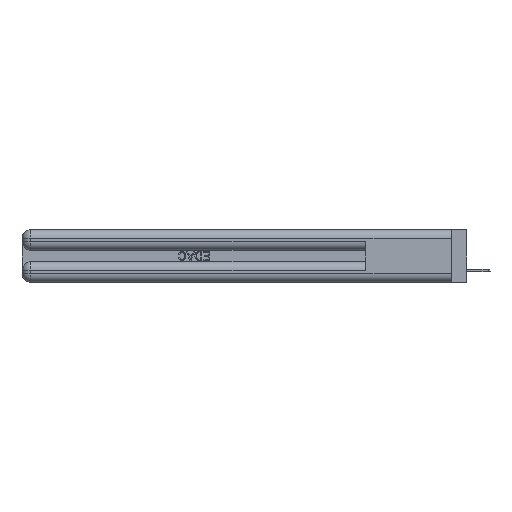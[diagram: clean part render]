
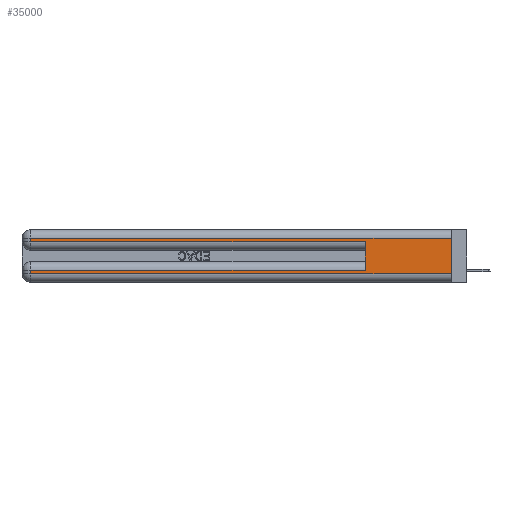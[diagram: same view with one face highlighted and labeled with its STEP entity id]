
A CAD part, left-side view. The second image highlights one B-rep face of the part: STEP entity #35000.
In plain terms, the highlighted planar face has unit normal (-1, 0, 0).
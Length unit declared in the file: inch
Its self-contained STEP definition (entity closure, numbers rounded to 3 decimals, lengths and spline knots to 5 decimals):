
#63 = ORIENTED_EDGE ( 'NONE', *, *, #6155, .F. ) ;
#1035 = DIRECTION ( 'NONE',  ( 0., -1., 0. ) ) ;
#2873 = FACE_OUTER_BOUND ( 'NONE', #14043, .T. ) ;
#3079 = DIRECTION ( 'NONE',  ( 0., 0., 1. ) ) ;
#4505 = LINE ( 'NONE', #20849, #42558 ) ;
#4718 = VERTEX_POINT ( 'NONE', #31403 ) ;
#4938 = LINE ( 'NONE', #20452, #36094 ) ;
#6155 = EDGE_CURVE ( 'NONE', #16280, #14997, #4505, .T. ) ;
#6618 = VERTEX_POINT ( 'NONE', #38588 ) ;
#6661 = CARTESIAN_POINT ( 'NONE',  ( 0., 0.6, 0.145 ) ) ;
#6908 = VERTEX_POINT ( 'NONE', #19527 ) ;
#7484 = LINE ( 'NONE', #41129, #29659 ) ;
#7557 = VECTOR ( 'NONE', #22286, 39.37008 ) ;
#7573 = LINE ( 'NONE', #6661, #22353 ) ;
#8105 = ORIENTED_EDGE ( 'NONE', *, *, #33060, .F. ) ;
#9645 = CARTESIAN_POINT ( 'NONE',  ( 0., 2.94, 0.085 ) ) ;
#10424 = DIRECTION ( 'NONE',  ( 1., 0., 0. ) ) ;
#10462 = CARTESIAN_POINT ( 'NONE',  ( 0., 0., 0.31 ) ) ;
#11125 = EDGE_CURVE ( 'NONE', #6908, #14997, #28765, .T. ) ;
#12103 = CARTESIAN_POINT ( 'NONE',  ( 0., 0., 0.31 ) ) ;
#14043 = EDGE_LOOP ( 'NONE', ( #63, #25486, #31046, #39941, #8105, #18049, #36142, #43435 ) ) ;
#14336 = CARTESIAN_POINT ( 'NONE',  ( 0., 2.94, 0.285 ) ) ;
#14997 = VERTEX_POINT ( 'NONE', #36721 ) ;
#16280 = VERTEX_POINT ( 'NONE', #10462 ) ;
#17372 = EDGE_CURVE ( 'NONE', #18128, #6908, #19222, .T. ) ;
#18049 = ORIENTED_EDGE ( 'NONE', *, *, #22112, .T. ) ;
#18128 = VERTEX_POINT ( 'NONE', #9645 ) ;
#19222 = LINE ( 'NONE', #38203, #41896 ) ;
#19527 = CARTESIAN_POINT ( 'NONE',  ( 0., 2.94, 0.06 ) ) ;
#20452 = CARTESIAN_POINT ( 'NONE',  ( 0., 2.94, 0.37 ) ) ;
#20581 = VERTEX_POINT ( 'NONE', #38969 ) ;
#20849 = CARTESIAN_POINT ( 'NONE',  ( 0., 0., 0.37 ) ) ;
#21319 = DIRECTION ( 'NONE',  ( 0., -1., 0. ) ) ;
#22112 = EDGE_CURVE ( 'NONE', #4718, #18128, #7484, .T. ) ;
#22286 = DIRECTION ( 'NONE',  ( 0., 1., 0. ) ) ;
#22353 = VECTOR ( 'NONE', #3079, 39.37008 ) ;
#22427 = VECTOR ( 'NONE', #1035, 39.37008 ) ;
#24831 = DIRECTION ( 'NONE',  ( 0., 0., -1. ) ) ;
#25486 = ORIENTED_EDGE ( 'NONE', *, *, #36674, .T. ) ;
#26225 = EDGE_CURVE ( 'NONE', #6618, #30972, #4938, .T. ) ;
#26374 = EDGE_CURVE ( 'NONE', #30972, #20581, #29264, .T. ) ;
#27460 = CARTESIAN_POINT ( 'NONE',  ( 0., 0., 0.06 ) ) ;
#28765 = LINE ( 'NONE', #27460, #22427 ) ;
#29264 = LINE ( 'NONE', #31600, #39817 ) ;
#29659 = VECTOR ( 'NONE', #40976, 39.37008 ) ;
#30433 = CARTESIAN_POINT ( 'NONE',  ( 0., 0., 0.37 ) ) ;
#30968 = DIRECTION ( 'NONE',  ( 0., 0., -1. ) ) ;
#30972 = VERTEX_POINT ( 'NONE', #14336 ) ;
#31046 = ORIENTED_EDGE ( 'NONE', *, *, #26225, .T. ) ;
#31403 = CARTESIAN_POINT ( 'NONE',  ( 0., 0.6, 0.085 ) ) ;
#31600 = CARTESIAN_POINT ( 'NONE',  ( 0., 0., 0.285 ) ) ;
#33060 = EDGE_CURVE ( 'NONE', #4718, #20581, #7573, .T. ) ;
#33829 = PLANE ( 'NONE',  #39838 ) ;
#33992 = DIRECTION ( 'NONE',  ( 0., 0., -1. ) ) ;
#35000 = ADVANCED_FACE ( 'NONE', ( #2873 ), #33829, .F. ) ;
#36094 = VECTOR ( 'NONE', #33992, 39.37008 ) ;
#36142 = ORIENTED_EDGE ( 'NONE', *, *, #17372, .T. ) ;
#36674 = EDGE_CURVE ( 'NONE', #16280, #6618, #42406, .T. ) ;
#36721 = CARTESIAN_POINT ( 'NONE',  ( 0., 0., 0.06 ) ) ;
#37222 = DIRECTION ( 'NONE',  ( 0., 0., -1. ) ) ;
#38203 = CARTESIAN_POINT ( 'NONE',  ( 0., 2.94, 0.37 ) ) ;
#38588 = CARTESIAN_POINT ( 'NONE',  ( 0., 2.94, 0.31 ) ) ;
#38969 = CARTESIAN_POINT ( 'NONE',  ( 0., 0.6, 0.285 ) ) ;
#39817 = VECTOR ( 'NONE', #21319, 39.37008 ) ;
#39838 = AXIS2_PLACEMENT_3D ( 'NONE', #30433, #10424, #37222 ) ;
#39941 = ORIENTED_EDGE ( 'NONE', *, *, #26374, .T. ) ;
#40976 = DIRECTION ( 'NONE',  ( 0., 1., 0. ) ) ;
#41129 = CARTESIAN_POINT ( 'NONE',  ( 0., 0., 0.085 ) ) ;
#41896 = VECTOR ( 'NONE', #30968, 39.37008 ) ;
#42406 = LINE ( 'NONE', #12103, #7557 ) ;
#42558 = VECTOR ( 'NONE', #24831, 39.37008 ) ;
#43435 = ORIENTED_EDGE ( 'NONE', *, *, #11125, .T. ) ;
